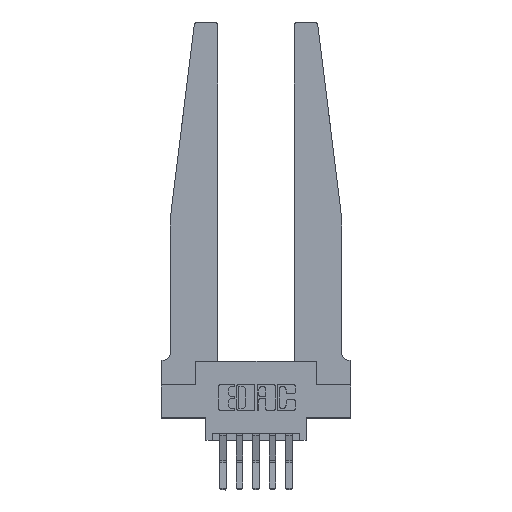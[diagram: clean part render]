
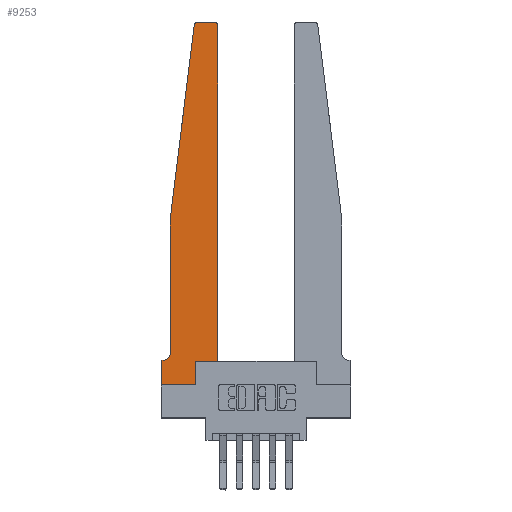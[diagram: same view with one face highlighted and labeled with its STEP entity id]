
A CAD part, top view. The second image highlights one B-rep face of the part: STEP entity #9253.
In plain terms, the highlighted planar face has unit normal (0, 0, 1).
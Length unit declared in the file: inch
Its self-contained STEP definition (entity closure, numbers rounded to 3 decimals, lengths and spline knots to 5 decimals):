
#9 = CARTESIAN_POINT ( 'NONE',  ( 0.065, 1.25, 0.37 ) ) ;
#51 = CARTESIAN_POINT ( 'NONE',  ( 0.065, 1.25, 0.37 ) ) ;
#87 = VERTEX_POINT ( 'NONE', #51 ) ;
#252 = CARTESIAN_POINT ( 'NONE',  ( 0.015, 0.1875, 0.37 ) ) ;
#264 = ORIENTED_EDGE ( 'NONE', *, *, #2075, .T. ) ;
#310 = VERTEX_POINT ( 'NONE', #2035 ) ;
#367 = EDGE_CURVE ( 'NONE', #4041, #3448, #9702, .T. ) ;
#527 = VERTEX_POINT ( 'NONE', #4824 ) ;
#779 = CARTESIAN_POINT ( 'NONE',  ( 0.395, 2.72, 0.37 ) ) ;
#846 = AXIS2_PLACEMENT_3D ( 'NONE', #10939, #2856, #9994 ) ;
#1000 = CARTESIAN_POINT ( 'NONE',  ( 0.015, 0.2375, 0.37 ) ) ;
#1003 = EDGE_CURVE ( 'NONE', #9603, #5020, #9395, .T. ) ;
#1101 = LINE ( 'NONE', #8353, #3904 ) ;
#1150 = CIRCLE ( 'NONE', #3170, 0.03 ) ;
#1202 = DIRECTION ( 'NONE',  ( 0., 1., 0. ) ) ;
#1327 = VECTOR ( 'NONE', #1202, 39.37008 ) ;
#1378 = VECTOR ( 'NONE', #3964, 39.37008 ) ;
#1396 = ORIENTED_EDGE ( 'NONE', *, *, #1003, .T. ) ;
#1488 = CARTESIAN_POINT ( 'NONE',  ( 0., 0., 0.37 ) ) ;
#1522 = EDGE_CURVE ( 'NONE', #7836, #9603, #1821, .T. ) ;
#1530 = AXIS2_PLACEMENT_3D ( 'NONE', #1000, #8240, #2066 ) ;
#1792 = PLANE ( 'NONE',  #846 ) ;
#1821 = LINE ( 'NONE', #13079, #6693 ) ;
#1841 = DIRECTION ( 'NONE',  ( 1., 0., 0. ) ) ;
#2035 = CARTESIAN_POINT ( 'NONE',  ( 0.065, 0.2375, 0.37 ) ) ;
#2054 = ORIENTED_EDGE ( 'NONE', *, *, #9353, .T. ) ;
#2066 = DIRECTION ( 'NONE',  ( -1., 0., 0. ) ) ;
#2073 = VERTEX_POINT ( 'NONE', #4956 ) ;
#2075 = EDGE_CURVE ( 'NONE', #2073, #3359, #1150, .T. ) ;
#2199 = ORIENTED_EDGE ( 'NONE', *, *, #7448, .T. ) ;
#2283 = ORIENTED_EDGE ( 'NONE', *, *, #11764, .T. ) ;
#2424 = EDGE_LOOP ( 'NONE', ( #2054, #12436, #2283, #2901, #3145, #11113, #7055, #10113, #10516, #1396, #2199, #264 ) ) ;
#2435 = VERTEX_POINT ( 'NONE', #252 ) ;
#2544 = DIRECTION ( 'NONE',  ( 1., 0., 0. ) ) ;
#2856 = DIRECTION ( 'NONE',  ( 0., 0., 1. ) ) ;
#2901 = ORIENTED_EDGE ( 'NONE', *, *, #12382, .T. ) ;
#3145 = ORIENTED_EDGE ( 'NONE', *, *, #6819, .T. ) ;
#3170 = AXIS2_PLACEMENT_3D ( 'NONE', #779, #8026, #1841 ) ;
#3179 = CARTESIAN_POINT ( 'NONE',  ( 0.425, 0.18, 0.37 ) ) ;
#3359 = VERTEX_POINT ( 'NONE', #9200 ) ;
#3400 = VERTEX_POINT ( 'NONE', #7250 ) ;
#3448 = VERTEX_POINT ( 'NONE', #11266 ) ;
#3518 = EDGE_CURVE ( 'NONE', #2435, #3400, #1101, .T. ) ;
#3904 = VECTOR ( 'NONE', #10382, 39.37008 ) ;
#3964 = DIRECTION ( 'NONE',  ( -0.122, -0.992, 0. ) ) ;
#3969 = VECTOR ( 'NONE', #5295, 39.37008 ) ;
#4041 = VERTEX_POINT ( 'NONE', #11735 ) ;
#4051 = EDGE_CURVE ( 'NONE', #3400, #527, #11008, .T. ) ;
#4176 = LINE ( 'NONE', #4966, #1378 ) ;
#4688 = CARTESIAN_POINT ( 'NONE',  ( 0., 0., 0.37 ) ) ;
#4824 = CARTESIAN_POINT ( 'NONE',  ( 0., 0., 0.37 ) ) ;
#4956 = CARTESIAN_POINT ( 'NONE',  ( 0.425, 2.72, 0.37 ) ) ;
#4966 = CARTESIAN_POINT ( 'NONE',  ( 0.065, 1.25, 0.37 ) ) ;
#5020 = VERTEX_POINT ( 'NONE', #3179 ) ;
#5295 = DIRECTION ( 'NONE',  ( 1., 0., 0. ) ) ;
#5988 = VECTOR ( 'NONE', #12726, 39.37008 ) ;
#6168 = DIRECTION ( 'NONE',  ( -1., 0., 0. ) ) ;
#6693 = VECTOR ( 'NONE', #10137, 39.37008 ) ;
#6819 = EDGE_CURVE ( 'NONE', #310, #2435, #8141, .T. ) ;
#7055 = ORIENTED_EDGE ( 'NONE', *, *, #4051, .T. ) ;
#7250 = CARTESIAN_POINT ( 'NONE',  ( 0., 0.1875, 0.37 ) ) ;
#7417 = CARTESIAN_POINT ( 'NONE',  ( 0.425, 0.18, 0.37 ) ) ;
#7435 = LINE ( 'NONE', #11163, #9786 ) ;
#7448 = EDGE_CURVE ( 'NONE', #5020, #2073, #11542, .T. ) ;
#7836 = VERTEX_POINT ( 'NONE', #10991 ) ;
#8026 = DIRECTION ( 'NONE',  ( 0., 0., 1. ) ) ;
#8079 = FACE_OUTER_BOUND ( 'NONE', #2424, .T. ) ;
#8141 = CIRCLE ( 'NONE', #1530, 0.05 ) ;
#8240 = DIRECTION ( 'NONE',  ( 0., 0., -1. ) ) ;
#8335 = DIRECTION ( 'NONE',  ( 0., -1., 0. ) ) ;
#8353 = CARTESIAN_POINT ( 'NONE',  ( 0.065, 0.1875, 0.37 ) ) ;
#8625 = LINE ( 'NONE', #9, #10963 ) ;
#9200 = CARTESIAN_POINT ( 'NONE',  ( 0.395, 2.75, 0.37 ) ) ;
#9253 = ADVANCED_FACE ( 'NONE', ( #8079 ), #1792, .T. ) ;
#9353 = EDGE_CURVE ( 'NONE', #3359, #4041, #7435, .T. ) ;
#9395 = LINE ( 'NONE', #11324, #3969 ) ;
#9574 = LINE ( 'NONE', #1488, #11895 ) ;
#9603 = VERTEX_POINT ( 'NONE', #12923 ) ;
#9702 = CIRCLE ( 'NONE', #10787, 0.03 ) ;
#9786 = VECTOR ( 'NONE', #6168, 39.37008 ) ;
#9994 = DIRECTION ( 'NONE',  ( 1., 0., 0. ) ) ;
#10113 = ORIENTED_EDGE ( 'NONE', *, *, #11517, .T. ) ;
#10137 = DIRECTION ( 'NONE',  ( 0., 1., 0. ) ) ;
#10382 = DIRECTION ( 'NONE',  ( -1., 0., 0. ) ) ;
#10516 = ORIENTED_EDGE ( 'NONE', *, *, #1522, .T. ) ;
#10787 = AXIS2_PLACEMENT_3D ( 'NONE', #11403, #11444, #11561 ) ;
#10939 = CARTESIAN_POINT ( 'NONE',  ( 0., 0.1875, 0.37 ) ) ;
#10963 = VECTOR ( 'NONE', #8335, 39.37008 ) ;
#10991 = CARTESIAN_POINT ( 'NONE',  ( 0.2605, 0., 0.37 ) ) ;
#11008 = LINE ( 'NONE', #4688, #5988 ) ;
#11113 = ORIENTED_EDGE ( 'NONE', *, *, #3518, .T. ) ;
#11163 = CARTESIAN_POINT ( 'NONE',  ( 0.25, 2.75, 0.37 ) ) ;
#11266 = CARTESIAN_POINT ( 'NONE',  ( 0.24675, 2.72367, 0.37 ) ) ;
#11324 = CARTESIAN_POINT ( 'NONE',  ( 0.425, 0.18, 0.37 ) ) ;
#11403 = CARTESIAN_POINT ( 'NONE',  ( 0.27653, 2.72, 0.37 ) ) ;
#11444 = DIRECTION ( 'NONE',  ( 0., 0., 1. ) ) ;
#11517 = EDGE_CURVE ( 'NONE', #527, #7836, #9574, .T. ) ;
#11542 = LINE ( 'NONE', #7417, #1327 ) ;
#11561 = DIRECTION ( 'NONE',  ( 1., 0., 0. ) ) ;
#11735 = CARTESIAN_POINT ( 'NONE',  ( 0.27653, 2.75, 0.37 ) ) ;
#11764 = EDGE_CURVE ( 'NONE', #3448, #87, #4176, .T. ) ;
#11895 = VECTOR ( 'NONE', #2544, 39.37008 ) ;
#12382 = EDGE_CURVE ( 'NONE', #87, #310, #8625, .T. ) ;
#12436 = ORIENTED_EDGE ( 'NONE', *, *, #367, .T. ) ;
#12726 = DIRECTION ( 'NONE',  ( 0., -1., 0. ) ) ;
#12923 = CARTESIAN_POINT ( 'NONE',  ( 0.2605, 0.18, 0.37 ) ) ;
#13079 = CARTESIAN_POINT ( 'NONE',  ( 0.2605, 0.18, 0.37 ) ) ;
